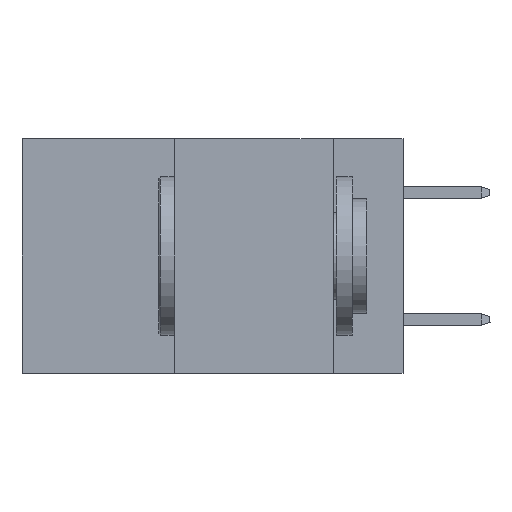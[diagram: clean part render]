
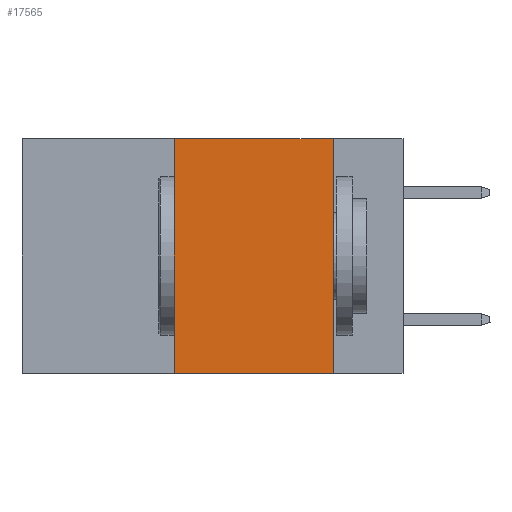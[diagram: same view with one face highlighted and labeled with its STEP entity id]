
A CAD part, left-side view. The second image highlights one B-rep face of the part: STEP entity #17565.
In plain terms, the highlighted planar face has unit normal (-1, 0, 0).
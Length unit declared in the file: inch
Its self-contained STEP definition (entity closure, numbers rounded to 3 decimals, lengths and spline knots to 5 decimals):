
#161 = EDGE_CURVE ( 'NONE', #2481, #13938, #16800, .T. ) ;
#503 = LINE ( 'NONE', #817, #10900 ) ;
#618 = ORIENTED_EDGE ( 'NONE', *, *, #161, .T. ) ;
#671 = ORIENTED_EDGE ( 'NONE', *, *, #10213, .F. ) ;
#817 = CARTESIAN_POINT ( 'NONE',  ( 0., 0.11, 0. ) ) ;
#1983 = DIRECTION ( 'NONE',  ( 0., 0., -1. ) ) ;
#2236 = VERTEX_POINT ( 'NONE', #13920 ) ;
#2324 = CARTESIAN_POINT ( 'NONE',  ( 0., 0.36, -0.37 ) ) ;
#2481 = VERTEX_POINT ( 'NONE', #2324 ) ;
#4359 = EDGE_CURVE ( 'NONE', #2236, #13938, #503, .T. ) ;
#4380 = EDGE_LOOP ( 'NONE', ( #5030, #671, #20592, #618 ) ) ;
#4964 = CARTESIAN_POINT ( 'NONE',  ( 0., 0.6, 0. ) ) ;
#5030 = ORIENTED_EDGE ( 'NONE', *, *, #4359, .F. ) ;
#6515 = DIRECTION ( 'NONE',  ( 0., 0., -1. ) ) ;
#6608 = VECTOR ( 'NONE', #16088, 39.37008 ) ;
#6864 = VECTOR ( 'NONE', #18585, 39.37008 ) ;
#8074 = LINE ( 'NONE', #16399, #6608 ) ;
#8537 = DIRECTION ( 'NONE',  ( 0., -1., 0. ) ) ;
#9706 = VECTOR ( 'NONE', #8537, 39.37008 ) ;
#10066 = PLANE ( 'NONE',  #10878 ) ;
#10213 = EDGE_CURVE ( 'NONE', #18821, #2236, #18119, .T. ) ;
#10651 = EDGE_CURVE ( 'NONE', #2481, #18821, #8074, .T. ) ;
#10878 = AXIS2_PLACEMENT_3D ( 'NONE', #14398, #16690, #6515 ) ;
#10900 = VECTOR ( 'NONE', #1983, 39.37008 ) ;
#13920 = CARTESIAN_POINT ( 'NONE',  ( 0., 0.11, 0. ) ) ;
#13938 = VERTEX_POINT ( 'NONE', #16915 ) ;
#14398 = CARTESIAN_POINT ( 'NONE',  ( 0., 0.6, 0. ) ) ;
#16088 = DIRECTION ( 'NONE',  ( 0., 0., 1. ) ) ;
#16399 = CARTESIAN_POINT ( 'NONE',  ( 0., 0.36, 0. ) ) ;
#16690 = DIRECTION ( 'NONE',  ( 1., 0., 0. ) ) ;
#16754 = CARTESIAN_POINT ( 'NONE',  ( 0., 0.36, 0. ) ) ;
#16800 = LINE ( 'NONE', #20146, #6864 ) ;
#16915 = CARTESIAN_POINT ( 'NONE',  ( 0., 0.11, -0.37 ) ) ;
#17565 = ADVANCED_FACE ( 'NONE', ( #19261 ), #10066, .F. ) ;
#18119 = LINE ( 'NONE', #4964, #9706 ) ;
#18585 = DIRECTION ( 'NONE',  ( 0., -1., 0. ) ) ;
#18821 = VERTEX_POINT ( 'NONE', #16754 ) ;
#19261 = FACE_OUTER_BOUND ( 'NONE', #4380, .T. ) ;
#20146 = CARTESIAN_POINT ( 'NONE',  ( 0., 0.6, -0.37 ) ) ;
#20592 = ORIENTED_EDGE ( 'NONE', *, *, #10651, .F. ) ;
